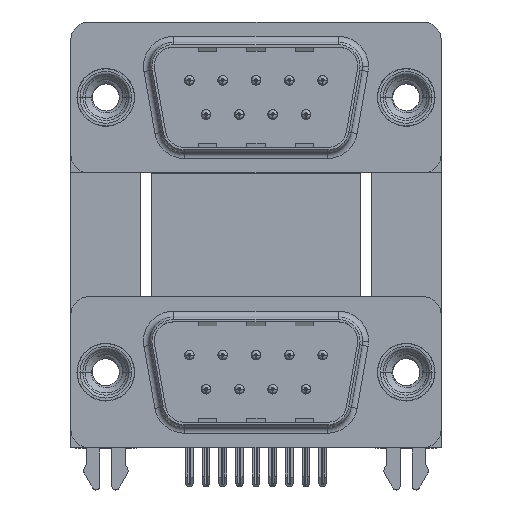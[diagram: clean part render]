
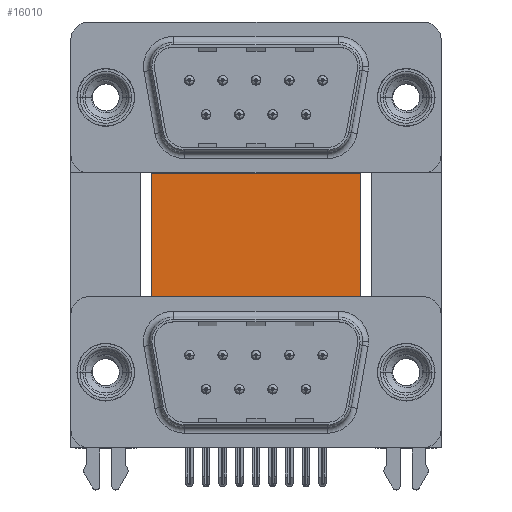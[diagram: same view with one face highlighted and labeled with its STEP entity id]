
A CAD part, top view. The second image highlights one B-rep face of the part: STEP entity #16010.
In plain terms, the highlighted planar face has unit normal (0, 0, 1).
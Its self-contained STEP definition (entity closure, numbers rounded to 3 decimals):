
#158 = LINE ( 'NONE', #11336, #22985 ) ;
#205 = VERTEX_POINT ( 'NONE', #10159 ) ;
#235 = ORIENTED_EDGE ( 'NONE', *, *, #22849, .T. ) ;
#284 = CARTESIAN_POINT ( 'NONE',  ( 22.09, -4.635, -12. ) ) ;
#346 = VECTOR ( 'NONE', #19794, 1000. ) ;
#366 = LINE ( 'NONE', #639, #13398 ) ;
#639 = CARTESIAN_POINT ( 'NONE',  ( 2.9, -3.735, -12. ) ) ;
#1101 = LINE ( 'NONE', #11309, #346 ) ;
#1429 = CARTESIAN_POINT ( 'NONE',  ( 2.4, -4.635, -12. ) ) ;
#1678 = ORIENTED_EDGE ( 'NONE', *, *, #15574, .T. ) ;
#2166 = LINE ( 'NONE', #25225, #24515 ) ;
#2436 = AXIS2_PLACEMENT_3D ( 'NONE', #9196, #17552, #25945 ) ;
#2826 = CARTESIAN_POINT ( 'NONE',  ( 3.79, -3.735, -12. ) ) ;
#3235 = CARTESIAN_POINT ( 'NONE',  ( 3.79, -0.735, -12. ) ) ;
#3534 = VECTOR ( 'NONE', #21395, 1000. ) ;
#3959 = CARTESIAN_POINT ( 'NONE',  ( 22.09, -3.735, -12. ) ) ;
#4013 = VECTOR ( 'NONE', #17335, 1000. ) ;
#4395 = LINE ( 'NONE', #6497, #14004 ) ;
#4632 = VERTEX_POINT ( 'NONE', #22259 ) ;
#5975 = ORIENTED_EDGE ( 'NONE', *, *, #10409, .T. ) ;
#6497 = CARTESIAN_POINT ( 'NONE',  ( 22.59, -4.635, -12. ) ) ;
#6681 = LINE ( 'NONE', #13095, #19785 ) ;
#6694 = ORIENTED_EDGE ( 'NONE', *, *, #9305, .F. ) ;
#7318 = DIRECTION ( 'NONE',  ( 1., 0., 0. ) ) ;
#8673 = EDGE_CURVE ( 'NONE', #24953, #25601, #366, .T. ) ;
#8876 = CARTESIAN_POINT ( 'NONE',  ( 3.79, 16.585, -12. ) ) ;
#9122 = DIRECTION ( 'NONE',  ( 1., 0., 0. ) ) ;
#9196 = CARTESIAN_POINT ( 'NONE',  ( 3.79, 16.585, -12. ) ) ;
#9305 = EDGE_CURVE ( 'NONE', #20462, #4632, #12724, .T. ) ;
#9421 = ORIENTED_EDGE ( 'NONE', *, *, #15890, .T. ) ;
#9585 = ORIENTED_EDGE ( 'NONE', *, *, #12222, .T. ) ;
#10159 = CARTESIAN_POINT ( 'NONE',  ( 22.59, -4.635, -12. ) ) ;
#10409 = EDGE_CURVE ( 'NONE', #205, #4632, #4395, .T. ) ;
#11070 = VERTEX_POINT ( 'NONE', #284 ) ;
#11133 = VERTEX_POINT ( 'NONE', #3235 ) ;
#11309 = CARTESIAN_POINT ( 'NONE',  ( 3.79, 16.585, -12. ) ) ;
#11335 = LINE ( 'NONE', #24046, #4013 ) ;
#11336 = CARTESIAN_POINT ( 'NONE',  ( 22.09, -4.635, -12. ) ) ;
#12222 = EDGE_CURVE ( 'NONE', #11070, #205, #158, .T. ) ;
#12724 = LINE ( 'NONE', #18722, #17095 ) ;
#13095 = CARTESIAN_POINT ( 'NONE',  ( 22.09, -3.735, -12. ) ) ;
#13098 = DIRECTION ( 'NONE',  ( 0., 1., 0. ) ) ;
#13398 = VECTOR ( 'NONE', #13098, 1000. ) ;
#13435 = LINE ( 'NONE', #2826, #21784 ) ;
#14004 = VECTOR ( 'NONE', #19321, 1000. ) ;
#14709 = EDGE_LOOP ( 'NONE', ( #21827, #9421, #9585, #5975, #6694, #27458, #1678, #25688, #235, #24670 ) ) ;
#15041 = DIRECTION ( 'NONE',  ( 0., -1., 0. ) ) ;
#15574 = EDGE_CURVE ( 'NONE', #23014, #11133, #1101, .T. ) ;
#15890 = EDGE_CURVE ( 'NONE', #24250, #11070, #6681, .T. ) ;
#16010 = ADVANCED_FACE ( 'NONE', ( #17152 ), #23565, .F. ) ;
#16710 = CARTESIAN_POINT ( 'NONE',  ( 21.2, 16.585, -12. ) ) ;
#16713 = VERTEX_POINT ( 'NONE', #1429 ) ;
#17095 = VECTOR ( 'NONE', #25307, 1000. ) ;
#17152 = FACE_OUTER_BOUND ( 'NONE', #14709, .T. ) ;
#17335 = DIRECTION ( 'NONE',  ( 1., 0., 0. ) ) ;
#17498 = LINE ( 'NONE', #23507, #3534 ) ;
#17552 = DIRECTION ( 'NONE',  ( 0., 0., -1. ) ) ;
#17921 = CARTESIAN_POINT ( 'NONE',  ( 2.9, -3.735, -12. ) ) ;
#18722 = CARTESIAN_POINT ( 'NONE',  ( 21.2, 16.585, -12. ) ) ;
#19321 = DIRECTION ( 'NONE',  ( -0.336, 0.942, 0. ) ) ;
#19785 = VECTOR ( 'NONE', #15041, 1000. ) ;
#19794 = DIRECTION ( 'NONE',  ( 0., -1., 0. ) ) ;
#20462 = VERTEX_POINT ( 'NONE', #16710 ) ;
#21395 = DIRECTION ( 'NONE',  ( -0.336, -0.942, 0. ) ) ;
#21784 = VECTOR ( 'NONE', #7318, 1000. ) ;
#21827 = ORIENTED_EDGE ( 'NONE', *, *, #25996, .T. ) ;
#22259 = CARTESIAN_POINT ( 'NONE',  ( 21.2, -0.735, -12. ) ) ;
#22849 = EDGE_CURVE ( 'NONE', #16713, #24953, #2166, .T. ) ;
#22977 = DIRECTION ( 'NONE',  ( 1., 0., 0. ) ) ;
#22985 = VECTOR ( 'NONE', #9122, 1000. ) ;
#23014 = VERTEX_POINT ( 'NONE', #8876 ) ;
#23300 = EDGE_CURVE ( 'NONE', #23014, #20462, #11335, .T. ) ;
#23507 = CARTESIAN_POINT ( 'NONE',  ( 2.4, -4.635, -12. ) ) ;
#23565 = PLANE ( 'NONE',  #2436 ) ;
#24046 = CARTESIAN_POINT ( 'NONE',  ( 3.79, 16.585, -12. ) ) ;
#24250 = VERTEX_POINT ( 'NONE', #3959 ) ;
#24515 = VECTOR ( 'NONE', #22977, 1000. ) ;
#24595 = CARTESIAN_POINT ( 'NONE',  ( 2.9, -4.635, -12. ) ) ;
#24670 = ORIENTED_EDGE ( 'NONE', *, *, #8673, .T. ) ;
#24953 = VERTEX_POINT ( 'NONE', #24595 ) ;
#25225 = CARTESIAN_POINT ( 'NONE',  ( 2.9, -4.635, -12. ) ) ;
#25307 = DIRECTION ( 'NONE',  ( 0., -1., 0. ) ) ;
#25601 = VERTEX_POINT ( 'NONE', #17921 ) ;
#25688 = ORIENTED_EDGE ( 'NONE', *, *, #27597, .T. ) ;
#25945 = DIRECTION ( 'NONE',  ( -1., 0., 0. ) ) ;
#25996 = EDGE_CURVE ( 'NONE', #25601, #24250, #13435, .T. ) ;
#27458 = ORIENTED_EDGE ( 'NONE', *, *, #23300, .F. ) ;
#27597 = EDGE_CURVE ( 'NONE', #11133, #16713, #17498, .T. ) ;
